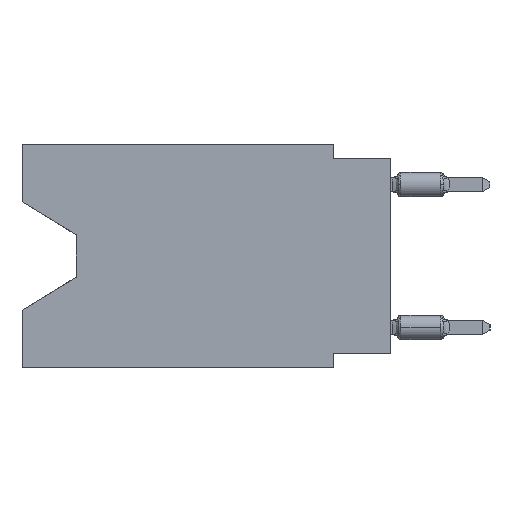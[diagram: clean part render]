
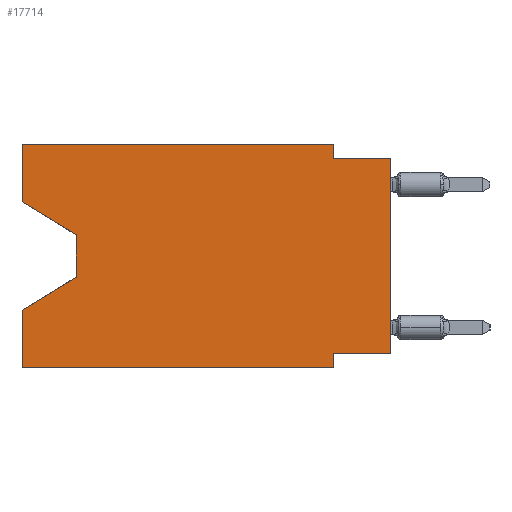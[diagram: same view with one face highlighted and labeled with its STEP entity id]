
A CAD part, left-side view. The second image highlights one B-rep face of the part: STEP entity #17714.
In plain terms, the highlighted planar face has unit normal (-1, 0, 0).
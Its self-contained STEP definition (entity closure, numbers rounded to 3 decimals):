
#628 = ORIENTED_EDGE ( 'NONE', *, *, #46944, .T. ) ;
#2310 = DIRECTION ( 'NONE',  ( 0., -0.855, -0.519 ) ) ;
#3267 = EDGE_CURVE ( 'NONE', #28725, #16515, #18317, .T. ) ;
#5252 = CARTESIAN_POINT ( 'NONE',  ( 0., 0., -9.271 ) ) ;
#5426 = CARTESIAN_POINT ( 'NONE',  ( 0., 13.97, -5.893 ) ) ;
#5951 = ORIENTED_EDGE ( 'NONE', *, *, #22034, .F. ) ;
#6153 = CARTESIAN_POINT ( 'NONE',  ( 0., 16.383, 0. ) ) ;
#6965 = DIRECTION ( 'NONE',  ( 0., 1., 0. ) ) ;
#7261 = CARTESIAN_POINT ( 'NONE',  ( 0., 13.97, -4.013 ) ) ;
#7390 = VERTEX_POINT ( 'NONE', #5252 ) ;
#7757 = ORIENTED_EDGE ( 'NONE', *, *, #50705, .F. ) ;
#8492 = ORIENTED_EDGE ( 'NONE', *, *, #14318, .F. ) ;
#8516 = VERTEX_POINT ( 'NONE', #34275 ) ;
#9490 = ORIENTED_EDGE ( 'NONE', *, *, #22745, .T. ) ;
#9922 = VERTEX_POINT ( 'NONE', #26377 ) ;
#10625 = EDGE_CURVE ( 'NONE', #36429, #36698, #17177, .T. ) ;
#11336 = CARTESIAN_POINT ( 'NONE',  ( 0., 16.383, -9.906 ) ) ;
#12173 = VERTEX_POINT ( 'NONE', #23904 ) ;
#12250 = LINE ( 'NONE', #33902, #25163 ) ;
#13746 = AXIS2_PLACEMENT_3D ( 'NONE', #55477, #15121, #32989 ) ;
#14227 = LINE ( 'NONE', #5426, #57560 ) ;
#14318 = EDGE_CURVE ( 'NONE', #40735, #16515, #19387, .T. ) ;
#14465 = VERTEX_POINT ( 'NONE', #49409 ) ;
#15121 = DIRECTION ( 'NONE',  ( 1., 0., 0. ) ) ;
#16515 = VERTEX_POINT ( 'NONE', #35796 ) ;
#17177 = LINE ( 'NONE', #35616, #26305 ) ;
#17524 = DIRECTION ( 'NONE',  ( 0., 0., -1. ) ) ;
#17639 = VECTOR ( 'NONE', #42151, 1000. ) ;
#17714 = ADVANCED_FACE ( 'NONE', ( #23908 ), #41743, .F. ) ;
#18317 = LINE ( 'NONE', #44948, #31739 ) ;
#19161 = CARTESIAN_POINT ( 'NONE',  ( 0., 2.54, 0. ) ) ;
#19387 = LINE ( 'NONE', #55069, #20298 ) ;
#20180 = CARTESIAN_POINT ( 'NONE',  ( 0., 16.383, -2.546 ) ) ;
#20298 = VECTOR ( 'NONE', #17524, 1000. ) ;
#20398 = EDGE_CURVE ( 'NONE', #7390, #40735, #12250, .T. ) ;
#22034 = EDGE_CURVE ( 'NONE', #36698, #14465, #47873, .T. ) ;
#22745 = EDGE_CURVE ( 'NONE', #12173, #8516, #42408, .T. ) ;
#23904 = CARTESIAN_POINT ( 'NONE',  ( 0., 16.383, -2.546 ) ) ;
#23908 = FACE_OUTER_BOUND ( 'NONE', #39651, .T. ) ;
#25163 = VECTOR ( 'NONE', #6965, 1000. ) ;
#25326 = EDGE_CURVE ( 'NONE', #14465, #34468, #45942, .T. ) ;
#26305 = VECTOR ( 'NONE', #53436, 1000. ) ;
#26377 = CARTESIAN_POINT ( 'NONE',  ( 0., 13.97, -5.893 ) ) ;
#28725 = VERTEX_POINT ( 'NONE', #11336 ) ;
#29507 = VECTOR ( 'NONE', #44741, 1000. ) ;
#29738 = CARTESIAN_POINT ( 'NONE',  ( 0., 16.383, 0. ) ) ;
#30151 = VECTOR ( 'NONE', #2310, 1000. ) ;
#30401 = LINE ( 'NONE', #7261, #55143 ) ;
#30947 = DIRECTION ( 'NONE',  ( 0., 0.855, -0.519 ) ) ;
#31217 = DIRECTION ( 'NONE',  ( 0., -1., 0. ) ) ;
#31288 = ORIENTED_EDGE ( 'NONE', *, *, #3267, .T. ) ;
#31659 = CARTESIAN_POINT ( 'NONE',  ( 0., 0., -0.635 ) ) ;
#31739 = VECTOR ( 'NONE', #31217, 1000. ) ;
#32989 = DIRECTION ( 'NONE',  ( 0., 0., -1. ) ) ;
#33136 = CARTESIAN_POINT ( 'NONE',  ( 0., 16.383, -7.36 ) ) ;
#33527 = ORIENTED_EDGE ( 'NONE', *, *, #20398, .F. ) ;
#33902 = CARTESIAN_POINT ( 'NONE',  ( 0., 0., -9.271 ) ) ;
#34275 = CARTESIAN_POINT ( 'NONE',  ( 0., 13.97, -4.013 ) ) ;
#34360 = ORIENTED_EDGE ( 'NONE', *, *, #46091, .T. ) ;
#34468 = VERTEX_POINT ( 'NONE', #52136 ) ;
#35616 = CARTESIAN_POINT ( 'NONE',  ( 0., 16.383, 0. ) ) ;
#35756 = CARTESIAN_POINT ( 'NONE',  ( 0., 2.54, -9.271 ) ) ;
#35796 = CARTESIAN_POINT ( 'NONE',  ( 0., 2.54, -9.906 ) ) ;
#35983 = EDGE_CURVE ( 'NONE', #8516, #9922, #30401, .T. ) ;
#36332 = DIRECTION ( 'NONE',  ( 0., -1., 0. ) ) ;
#36429 = VERTEX_POINT ( 'NONE', #29738 ) ;
#36698 = VERTEX_POINT ( 'NONE', #19161 ) ;
#37769 = LINE ( 'NONE', #6153, #17639 ) ;
#38232 = CARTESIAN_POINT ( 'NONE',  ( 0., 2.54, 0. ) ) ;
#38583 = DIRECTION ( 'NONE',  ( 0., 0., -1. ) ) ;
#39136 = VERTEX_POINT ( 'NONE', #33136 ) ;
#39313 = CARTESIAN_POINT ( 'NONE',  ( 0., 16.383, 0. ) ) ;
#39651 = EDGE_LOOP ( 'NONE', ( #9490, #48356, #628, #7757, #31288, #8492, #33527, #34360, #54588, #5951, #52380, #40554 ) ) ;
#40554 = ORIENTED_EDGE ( 'NONE', *, *, #43997, .F. ) ;
#40735 = VERTEX_POINT ( 'NONE', #35756 ) ;
#41743 = PLANE ( 'NONE',  #13746 ) ;
#42151 = DIRECTION ( 'NONE',  ( 0., 0., 1. ) ) ;
#42408 = LINE ( 'NONE', #20180, #30151 ) ;
#43200 = VECTOR ( 'NONE', #43787, 1000. ) ;
#43787 = DIRECTION ( 'NONE',  ( 0., 0., -1. ) ) ;
#43997 = EDGE_CURVE ( 'NONE', #12173, #36429, #52751, .T. ) ;
#44741 = DIRECTION ( 'NONE',  ( 0., 0., 1. ) ) ;
#44948 = CARTESIAN_POINT ( 'NONE',  ( 0., 16.383, -9.906 ) ) ;
#45942 = LINE ( 'NONE', #31659, #49871 ) ;
#46091 = EDGE_CURVE ( 'NONE', #7390, #34468, #54089, .T. ) ;
#46944 = EDGE_CURVE ( 'NONE', #9922, #39136, #14227, .T. ) ;
#47084 = VECTOR ( 'NONE', #48081, 1000. ) ;
#47873 = LINE ( 'NONE', #38232, #43200 ) ;
#48081 = DIRECTION ( 'NONE',  ( 0., 0., 1. ) ) ;
#48356 = ORIENTED_EDGE ( 'NONE', *, *, #35983, .T. ) ;
#49409 = CARTESIAN_POINT ( 'NONE',  ( 0., 2.54, -0.635 ) ) ;
#49871 = VECTOR ( 'NONE', #36332, 1000. ) ;
#50705 = EDGE_CURVE ( 'NONE', #28725, #39136, #37769, .T. ) ;
#52136 = CARTESIAN_POINT ( 'NONE',  ( 0., 0., -0.635 ) ) ;
#52380 = ORIENTED_EDGE ( 'NONE', *, *, #10625, .F. ) ;
#52751 = LINE ( 'NONE', #39313, #47084 ) ;
#53436 = DIRECTION ( 'NONE',  ( 0., -1., 0. ) ) ;
#53509 = CARTESIAN_POINT ( 'NONE',  ( 0., 0., 0. ) ) ;
#54089 = LINE ( 'NONE', #53509, #29507 ) ;
#54588 = ORIENTED_EDGE ( 'NONE', *, *, #25326, .F. ) ;
#55069 = CARTESIAN_POINT ( 'NONE',  ( 0., 2.54, -9.906 ) ) ;
#55143 = VECTOR ( 'NONE', #38583, 1000. ) ;
#55477 = CARTESIAN_POINT ( 'NONE',  ( 0., 16.383, 0. ) ) ;
#57560 = VECTOR ( 'NONE', #30947, 1000. ) ;
